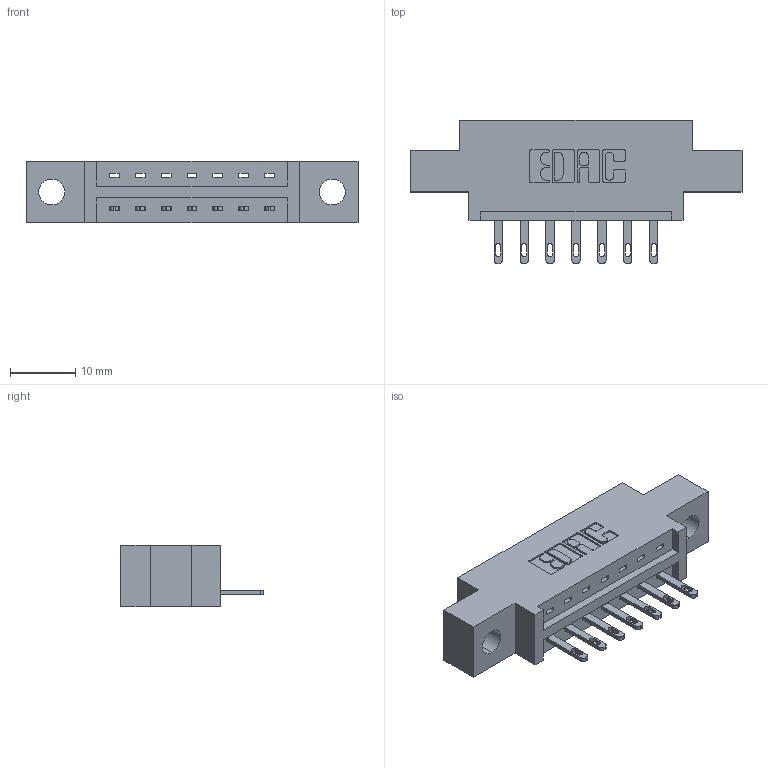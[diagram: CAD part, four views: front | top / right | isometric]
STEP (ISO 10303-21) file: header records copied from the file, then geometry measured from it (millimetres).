
FILE_DESCRIPTION (( 'STEP AP203' ), '1' );
FILE_NAME ('337-007-500-604.STEP', '2018-08-03T19:39:07', ( '' ), ( '' ), 'SwSTEP 2.0', 'SolidWorks 2016', '' );
FILE_SCHEMA (( 'CONFIG_CONTROL_DESIGN' ));
Length unit declared in the file: inch
Products named in the file (3): 337-007-500-604; 337 Part_0.170 Offset - 0.156 Dia-TH; 345-292-001_345-293-100
Assembly tree (8 placements, depth 2):
  337-007-500-604
    337 Part_0.170 Offset - 0.156 Dia-TH
    345-292-001_345-293-100  x7
Bounding box: 50.75 x 21.85 x 9.4 mm (x, y, z)
Volume: 4635.5 mm3; surface area: 4503.9 mm2
Topology: 8 solids, 8 shells, 524 faces, 1583 edges, 1054 vertices
Faces by surface type: plane 354, cylinder 170
Entity records: 9795 total; most frequent: CARTESIAN_POINT 1711, ORIENTED_EDGE 1654, DIRECTION 1513, EDGE_CURVE 827, LINE 695, VECTOR 695, VERTEX_POINT 550, AXIS2_PLACEMENT_3D 409
